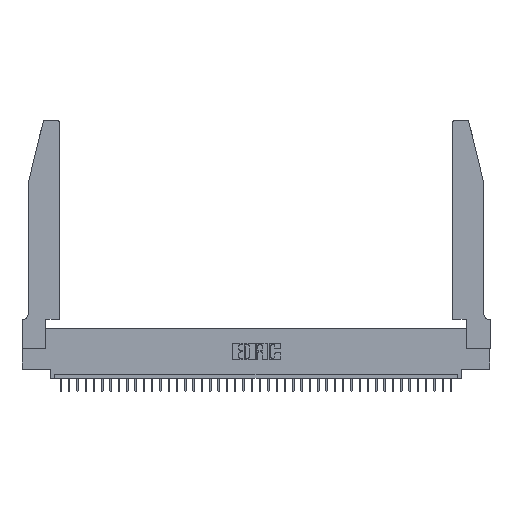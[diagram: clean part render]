
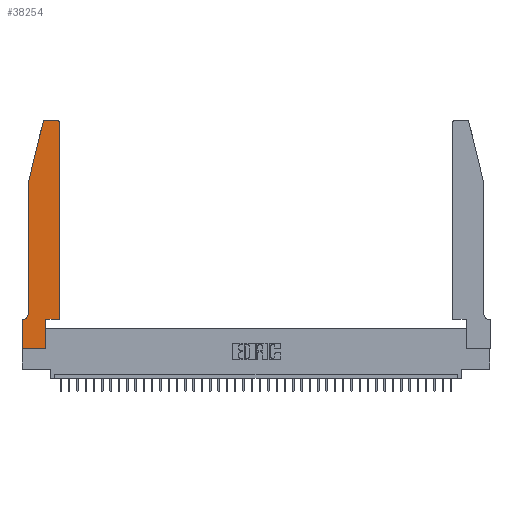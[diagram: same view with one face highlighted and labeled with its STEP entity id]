
A CAD part, top view. The second image highlights one B-rep face of the part: STEP entity #38254.
In plain terms, the highlighted planar face has unit normal (0, 0, 1).
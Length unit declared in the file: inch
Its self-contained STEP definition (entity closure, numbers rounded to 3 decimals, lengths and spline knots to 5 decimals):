
#58 = CIRCLE ( 'NONE', #22997, 0.03 ) ;
#733 = DIRECTION ( 'NONE',  ( 0., 1., 0. ) ) ;
#829 = CARTESIAN_POINT ( 'NONE',  ( 0.0055, 0.35, 0.37 ) ) ;
#1079 = DIRECTION ( 'NONE',  ( 0., -1., 0. ) ) ;
#1274 = CIRCLE ( 'NONE', #20077, 0.07 ) ;
#1539 = CARTESIAN_POINT ( 'NONE',  ( 0.2865, 0.35, 0.37 ) ) ;
#1862 = EDGE_CURVE ( 'NONE', #39241, #8091, #20116, .T. ) ;
#2095 = VECTOR ( 'NONE', #1079, 39.37008 ) ;
#2275 = CIRCLE ( 'NONE', #32464, 0.03 ) ;
#2401 = CARTESIAN_POINT ( 'NONE',  ( 0.2865, 0., 0.37 ) ) ;
#2464 = EDGE_CURVE ( 'NONE', #31086, #23949, #58, .T. ) ;
#2705 = DIRECTION ( 'NONE',  ( 1., 0., 0. ) ) ;
#2769 = DIRECTION ( 'NONE',  ( -0.239, -0.971, 0. ) ) ;
#2931 = CARTESIAN_POINT ( 'NONE',  ( 0.284, 2.72, 0.37 ) ) ;
#3038 = ORIENTED_EDGE ( 'NONE', *, *, #20144, .T. ) ;
#3797 = CARTESIAN_POINT ( 'NONE',  ( 0.0055, 0.42, 0.37 ) ) ;
#3844 = EDGE_CURVE ( 'NONE', #37949, #32126, #17978, .T. ) ;
#3881 = LINE ( 'NONE', #8132, #36503 ) ;
#4309 = VERTEX_POINT ( 'NONE', #30675 ) ;
#5107 = CARTESIAN_POINT ( 'NONE',  ( 0., 0.35, 0.37 ) ) ;
#5351 = DIRECTION ( 'NONE',  ( 0., -1., 0. ) ) ;
#5412 = CARTESIAN_POINT ( 'NONE',  ( 0.2605, 2.75, 0.37 ) ) ;
#5956 = FACE_OUTER_BOUND ( 'NONE', #26862, .T. ) ;
#6166 = ORIENTED_EDGE ( 'NONE', *, *, #28332, .T. ) ;
#7427 = LINE ( 'NONE', #35500, #2095 ) ;
#7938 = LINE ( 'NONE', #5412, #31743 ) ;
#8078 = VECTOR ( 'NONE', #28497, 39.37008 ) ;
#8091 = VERTEX_POINT ( 'NONE', #5107 ) ;
#8132 = CARTESIAN_POINT ( 'NONE',  ( 0., 0., 0.37 ) ) ;
#8146 = VERTEX_POINT ( 'NONE', #2401 ) ;
#8559 = DIRECTION ( 'NONE',  ( -1., 0., 0. ) ) ;
#9067 = EDGE_CURVE ( 'NONE', #24856, #8146, #3881, .T. ) ;
#9127 = VECTOR ( 'NONE', #2769, 39.37008 ) ;
#9307 = DIRECTION ( 'NONE',  ( 0., 0., 1. ) ) ;
#9565 = LINE ( 'NONE', #12149, #9127 ) ;
#9848 = VECTOR ( 'NONE', #37132, 39.37008 ) ;
#11646 = EDGE_CURVE ( 'NONE', #4309, #39241, #1274, .T. ) ;
#12149 = CARTESIAN_POINT ( 'NONE',  ( 0.0755, 2., 0.37 ) ) ;
#12557 = ORIENTED_EDGE ( 'NONE', *, *, #26112, .T. ) ;
#12777 = DIRECTION ( 'NONE',  ( -1., 0., 0. ) ) ;
#14706 = DIRECTION ( 'NONE',  ( 1., 0., 0. ) ) ;
#15120 = CARTESIAN_POINT ( 'NONE',  ( 0., 0.35, 0.37 ) ) ;
#15225 = EDGE_CURVE ( 'NONE', #8091, #24856, #7427, .T. ) ;
#15534 = CARTESIAN_POINT ( 'NONE',  ( 0.4505, 0.35, 0.37 ) ) ;
#17961 = PLANE ( 'NONE',  #33864 ) ;
#17978 = LINE ( 'NONE', #15534, #39366 ) ;
#18929 = CARTESIAN_POINT ( 'NONE',  ( 0.0755, 2., 0.37 ) ) ;
#19833 = EDGE_CURVE ( 'NONE', #8146, #37949, #40166, .T. ) ;
#20077 = AXIS2_PLACEMENT_3D ( 'NONE', #3797, #25170, #12777 ) ;
#20116 = LINE ( 'NONE', #39154, #9848 ) ;
#20144 = EDGE_CURVE ( 'NONE', #39116, #4309, #20697, .T. ) ;
#20239 = ORIENTED_EDGE ( 'NONE', *, *, #1862, .T. ) ;
#20697 = LINE ( 'NONE', #21001, #30449 ) ;
#21001 = CARTESIAN_POINT ( 'NONE',  ( 0.0755, 2., 0.37 ) ) ;
#21162 = ORIENTED_EDGE ( 'NONE', *, *, #11646, .T. ) ;
#21225 = DIRECTION ( 'NONE',  ( 1., 0., 0. ) ) ;
#21300 = ORIENTED_EDGE ( 'NONE', *, *, #3844, .T. ) ;
#21350 = CARTESIAN_POINT ( 'NONE',  ( 0.4205, 2.72, 0.37 ) ) ;
#22096 = CARTESIAN_POINT ( 'NONE',  ( 0.4505, 0.35, 0.37 ) ) ;
#22997 = AXIS2_PLACEMENT_3D ( 'NONE', #2931, #9307, #36956 ) ;
#23007 = CARTESIAN_POINT ( 'NONE',  ( 0.25487, 2.72718, 0.37 ) ) ;
#23949 = VERTEX_POINT ( 'NONE', #23007 ) ;
#24313 = LINE ( 'NONE', #22096, #33996 ) ;
#24470 = VERTEX_POINT ( 'NONE', #35891 ) ;
#24856 = VERTEX_POINT ( 'NONE', #30819 ) ;
#25153 = DIRECTION ( 'NONE',  ( 1., 0., 0. ) ) ;
#25170 = DIRECTION ( 'NONE',  ( 0., 0., -1. ) ) ;
#25684 = ORIENTED_EDGE ( 'NONE', *, *, #19833, .T. ) ;
#26112 = EDGE_CURVE ( 'NONE', #32126, #30448, #24313, .T. ) ;
#26862 = EDGE_LOOP ( 'NONE', ( #36557, #39871, #6166, #3038, #21162, #20239, #36925, #37704, #25684, #21300, #12557, #32864 ) ) ;
#28332 = EDGE_CURVE ( 'NONE', #23949, #39116, #9565, .T. ) ;
#28497 = DIRECTION ( 'NONE',  ( 0., 1., 0. ) ) ;
#28811 = CARTESIAN_POINT ( 'NONE',  ( 0.2865, 0.35, 0.37 ) ) ;
#28884 = EDGE_CURVE ( 'NONE', #30448, #24470, #2275, .T. ) ;
#30448 = VERTEX_POINT ( 'NONE', #34551 ) ;
#30449 = VECTOR ( 'NONE', #5351, 39.37008 ) ;
#30587 = DIRECTION ( 'NONE',  ( 0., 0., 1. ) ) ;
#30675 = CARTESIAN_POINT ( 'NONE',  ( 0.0755, 0.42, 0.37 ) ) ;
#30819 = CARTESIAN_POINT ( 'NONE',  ( 0., 0., 0.37 ) ) ;
#31086 = VERTEX_POINT ( 'NONE', #35422 ) ;
#31743 = VECTOR ( 'NONE', #8559, 39.37008 ) ;
#32126 = VERTEX_POINT ( 'NONE', #38445 ) ;
#32464 = AXIS2_PLACEMENT_3D ( 'NONE', #21350, #39675, #25153 ) ;
#32864 = ORIENTED_EDGE ( 'NONE', *, *, #28884, .T. ) ;
#33864 = AXIS2_PLACEMENT_3D ( 'NONE', #15120, #30587, #2705 ) ;
#33996 = VECTOR ( 'NONE', #733, 39.37008 ) ;
#34551 = CARTESIAN_POINT ( 'NONE',  ( 0.4505, 2.72, 0.37 ) ) ;
#35422 = CARTESIAN_POINT ( 'NONE',  ( 0.284, 2.75, 0.37 ) ) ;
#35500 = CARTESIAN_POINT ( 'NONE',  ( 0., 0., 0.37 ) ) ;
#35891 = CARTESIAN_POINT ( 'NONE',  ( 0.4205, 2.75, 0.37 ) ) ;
#36503 = VECTOR ( 'NONE', #14706, 39.37008 ) ;
#36557 = ORIENTED_EDGE ( 'NONE', *, *, #38344, .T. ) ;
#36925 = ORIENTED_EDGE ( 'NONE', *, *, #15225, .T. ) ;
#36956 = DIRECTION ( 'NONE',  ( 1., 0., 0. ) ) ;
#37132 = DIRECTION ( 'NONE',  ( -1., 0., 0. ) ) ;
#37704 = ORIENTED_EDGE ( 'NONE', *, *, #9067, .T. ) ;
#37949 = VERTEX_POINT ( 'NONE', #28811 ) ;
#38254 = ADVANCED_FACE ( 'NONE', ( #5956 ), #17961, .T. ) ;
#38344 = EDGE_CURVE ( 'NONE', #24470, #31086, #7938, .T. ) ;
#38445 = CARTESIAN_POINT ( 'NONE',  ( 0.4505, 0.35, 0.37 ) ) ;
#39116 = VERTEX_POINT ( 'NONE', #18929 ) ;
#39154 = CARTESIAN_POINT ( 'NONE',  ( 0.0755, 0.35, 0.37 ) ) ;
#39241 = VERTEX_POINT ( 'NONE', #829 ) ;
#39366 = VECTOR ( 'NONE', #21225, 39.37008 ) ;
#39675 = DIRECTION ( 'NONE',  ( 0., 0., 1. ) ) ;
#39871 = ORIENTED_EDGE ( 'NONE', *, *, #2464, .T. ) ;
#40166 = LINE ( 'NONE', #1539, #8078 ) ;
